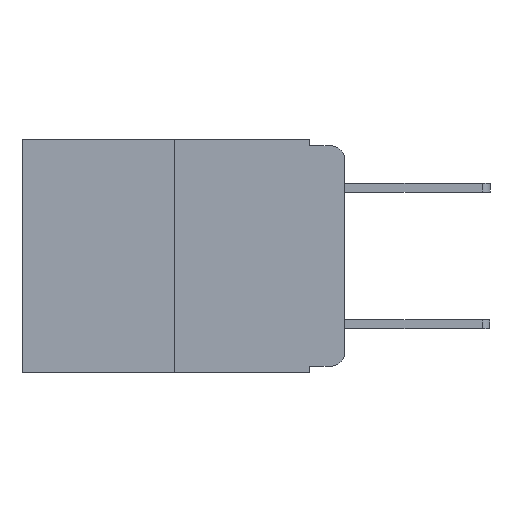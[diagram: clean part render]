
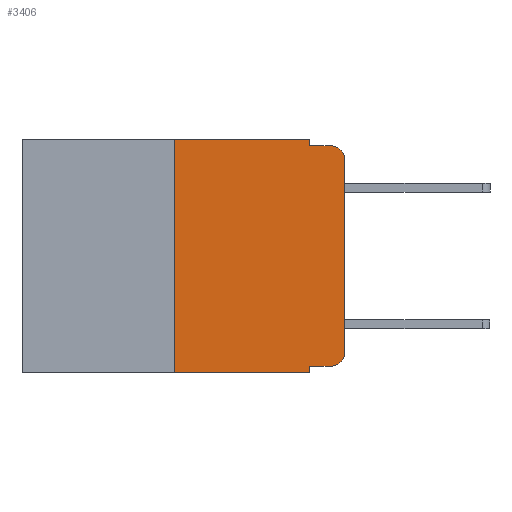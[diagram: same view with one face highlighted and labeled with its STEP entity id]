
A CAD part, left-side view. The second image highlights one B-rep face of the part: STEP entity #3406.
In plain terms, the highlighted planar face has unit normal (-1, 0, 0).
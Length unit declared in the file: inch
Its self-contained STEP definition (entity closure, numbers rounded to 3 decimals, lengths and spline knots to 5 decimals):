
#157 = VERTEX_POINT ( 'NONE', #17840 ) ;
#183 = EDGE_CURVE ( 'NONE', #5618, #6462, #12887, .T. ) ;
#648 = DIRECTION ( 'NONE',  ( 0., -1., 0. ) ) ;
#1082 = LINE ( 'NONE', #17815, #7939 ) ;
#1195 = ORIENTED_EDGE ( 'NONE', *, *, #16530, .F. ) ;
#1293 = EDGE_CURVE ( 'NONE', #5930, #6462, #7768, .T. ) ;
#1735 = LINE ( 'NONE', #2489, #16451 ) ;
#2384 = EDGE_CURVE ( 'NONE', #12648, #5930, #1082, .T. ) ;
#2489 = CARTESIAN_POINT ( 'NONE',  ( 0., 0.051, -0.333 ) ) ;
#2490 = CARTESIAN_POINT ( 'NONE',  ( 0., 0.051, -0.01 ) ) ;
#3270 = AXIS2_PLACEMENT_3D ( 'NONE', #14056, #5952, #15369 ) ;
#3284 = ORIENTED_EDGE ( 'NONE', *, *, #14898, .F. ) ;
#3406 = ADVANCED_FACE ( 'NONE', ( #17351 ), #17367, .F. ) ;
#4069 = CARTESIAN_POINT ( 'NONE',  ( 0., 0.473, -0.343 ) ) ;
#4251 = CARTESIAN_POINT ( 'NONE',  ( 0., 0.473, 0. ) ) ;
#4276 = EDGE_CURVE ( 'NONE', #6102, #4298, #13652, .T. ) ;
#4298 = VERTEX_POINT ( 'NONE', #16319 ) ;
#4383 = AXIS2_PLACEMENT_3D ( 'NONE', #7587, #7628, #7476 ) ;
#4723 = DIRECTION ( 'NONE',  ( 0., 0., 1. ) ) ;
#5098 = CIRCLE ( 'NONE', #3270, 0.02 ) ;
#5273 = DIRECTION ( 'NONE',  ( 0., 0., -1. ) ) ;
#5402 = VECTOR ( 'NONE', #5273, 39.37008 ) ;
#5618 = VERTEX_POINT ( 'NONE', #13427 ) ;
#5698 = ORIENTED_EDGE ( 'NONE', *, *, #2384, .T. ) ;
#5708 = DIRECTION ( 'NONE',  ( 0., -1., 0. ) ) ;
#5930 = VERTEX_POINT ( 'NONE', #7302 ) ;
#5952 = DIRECTION ( 'NONE',  ( -1., 0., 0. ) ) ;
#5995 = ORIENTED_EDGE ( 'NONE', *, *, #14769, .T. ) ;
#6102 = VERTEX_POINT ( 'NONE', #10303 ) ;
#6114 = CARTESIAN_POINT ( 'NONE',  ( 0., 0., -0.313 ) ) ;
#6462 = VERTEX_POINT ( 'NONE', #17578 ) ;
#6746 = ORIENTED_EDGE ( 'NONE', *, *, #1293, .T. ) ;
#7302 = CARTESIAN_POINT ( 'NONE',  ( 0., 0., -0.03 ) ) ;
#7476 = DIRECTION ( 'NONE',  ( 0., 0., -1. ) ) ;
#7587 = CARTESIAN_POINT ( 'NONE',  ( 0., 0.473, 0. ) ) ;
#7628 = DIRECTION ( 'NONE',  ( 1., 0., 0. ) ) ;
#7768 = CIRCLE ( 'NONE', #12380, 0.02 ) ;
#7939 = VECTOR ( 'NONE', #11293, 39.37008 ) ;
#8483 = DIRECTION ( 'NONE',  ( 0., 0., -1. ) ) ;
#8489 = DIRECTION ( 'NONE',  ( 0., 0., -1. ) ) ;
#9010 = DIRECTION ( 'NONE',  ( -1., 0., 0. ) ) ;
#9069 = LINE ( 'NONE', #14249, #16198 ) ;
#9252 = CARTESIAN_POINT ( 'NONE',  ( 0., 0.02, -0.03 ) ) ;
#9310 = VECTOR ( 'NONE', #8489, 39.37008 ) ;
#10095 = VECTOR ( 'NONE', #12290, 39.37008 ) ;
#10303 = CARTESIAN_POINT ( 'NONE',  ( 0., 0.25, -0.343 ) ) ;
#10390 = VERTEX_POINT ( 'NONE', #17927 ) ;
#10882 = ORIENTED_EDGE ( 'NONE', *, *, #15650, .F. ) ;
#10886 = DIRECTION ( 'NONE',  ( 0., -1., 0. ) ) ;
#11293 = DIRECTION ( 'NONE',  ( 0., 0., 1. ) ) ;
#11599 = CARTESIAN_POINT ( 'NONE',  ( 0., 0.051, 0. ) ) ;
#12202 = LINE ( 'NONE', #13386, #5402 ) ;
#12290 = DIRECTION ( 'NONE',  ( 0., -1., 0. ) ) ;
#12380 = AXIS2_PLACEMENT_3D ( 'NONE', #9252, #9010, #8483 ) ;
#12648 = VERTEX_POINT ( 'NONE', #6114 ) ;
#12885 = LINE ( 'NONE', #17888, #9310 ) ;
#12887 = LINE ( 'NONE', #2490, #15601 ) ;
#13386 = CARTESIAN_POINT ( 'NONE',  ( 0., 0.051, 0. ) ) ;
#13410 = VERTEX_POINT ( 'NONE', #11599 ) ;
#13427 = CARTESIAN_POINT ( 'NONE',  ( 0., 0.051, -0.01 ) ) ;
#13652 = LINE ( 'NONE', #4069, #10095 ) ;
#13864 = EDGE_CURVE ( 'NONE', #10390, #12648, #5098, .T. ) ;
#14056 = CARTESIAN_POINT ( 'NONE',  ( 0., 0.02, -0.313 ) ) ;
#14249 = CARTESIAN_POINT ( 'NONE',  ( 0., 0.25, 0. ) ) ;
#14389 = VECTOR ( 'NONE', #5708, 39.37008 ) ;
#14649 = ORIENTED_EDGE ( 'NONE', *, *, #13864, .T. ) ;
#14769 = EDGE_CURVE ( 'NONE', #17049, #10390, #1735, .T. ) ;
#14898 = EDGE_CURVE ( 'NONE', #157, #13410, #17947, .T. ) ;
#15201 = ORIENTED_EDGE ( 'NONE', *, *, #17464, .F. ) ;
#15369 = DIRECTION ( 'NONE',  ( 0., 0., -1. ) ) ;
#15443 = ORIENTED_EDGE ( 'NONE', *, *, #183, .F. ) ;
#15601 = VECTOR ( 'NONE', #648, 39.37008 ) ;
#15650 = EDGE_CURVE ( 'NONE', #17049, #4298, #12885, .T. ) ;
#16198 = VECTOR ( 'NONE', #4723, 39.37008 ) ;
#16319 = CARTESIAN_POINT ( 'NONE',  ( 0., 0.051, -0.343 ) ) ;
#16451 = VECTOR ( 'NONE', #10886, 39.37008 ) ;
#16530 = EDGE_CURVE ( 'NONE', #6102, #157, #9069, .T. ) ;
#16592 = CARTESIAN_POINT ( 'NONE',  ( 0., 0.051, -0.333 ) ) ;
#17049 = VERTEX_POINT ( 'NONE', #16592 ) ;
#17351 = FACE_OUTER_BOUND ( 'NONE', #17617, .T. ) ;
#17367 = PLANE ( 'NONE',  #4383 ) ;
#17464 = EDGE_CURVE ( 'NONE', #13410, #5618, #12202, .T. ) ;
#17578 = CARTESIAN_POINT ( 'NONE',  ( 0., 0.02, -0.01 ) ) ;
#17617 = EDGE_LOOP ( 'NONE', ( #5698, #6746, #15443, #15201, #3284, #1195, #17762, #10882, #5995, #14649 ) ) ;
#17762 = ORIENTED_EDGE ( 'NONE', *, *, #4276, .T. ) ;
#17815 = CARTESIAN_POINT ( 'NONE',  ( 0., 0., 0. ) ) ;
#17840 = CARTESIAN_POINT ( 'NONE',  ( 0., 0.25, 0. ) ) ;
#17888 = CARTESIAN_POINT ( 'NONE',  ( 0., 0.051, 0. ) ) ;
#17927 = CARTESIAN_POINT ( 'NONE',  ( 0., 0.02, -0.333 ) ) ;
#17947 = LINE ( 'NONE', #4251, #14389 ) ;
